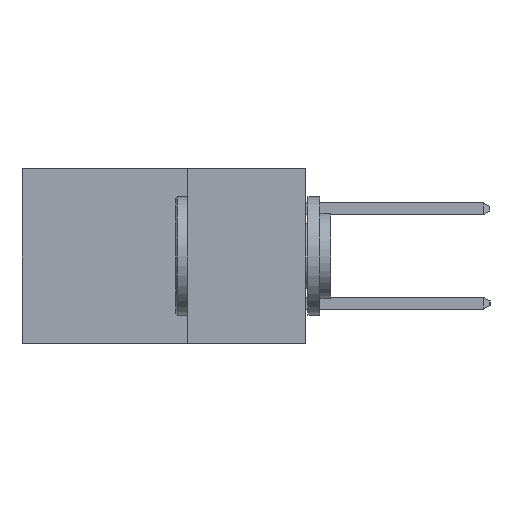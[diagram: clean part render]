
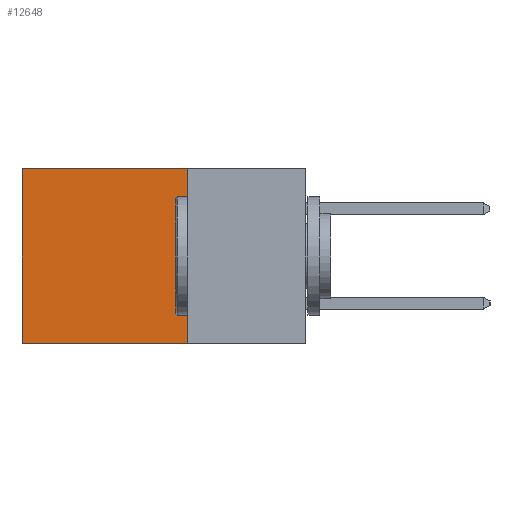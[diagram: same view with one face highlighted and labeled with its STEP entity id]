
A CAD part, left-side view. The second image highlights one B-rep face of the part: STEP entity #12648.
In plain terms, the highlighted planar face has unit normal (-1, 0, 0).
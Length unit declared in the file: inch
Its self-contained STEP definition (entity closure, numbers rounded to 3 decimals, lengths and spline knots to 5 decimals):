
#1976 = CARTESIAN_POINT ( 'NONE',  ( 0.2615, 0.25, -0.37 ) ) ;
#2145 = VECTOR ( 'NONE', #4501, 39.37008 ) ;
#2227 = CARTESIAN_POINT ( 'NONE',  ( 0.2615, 0.25, 0. ) ) ;
#4171 = DIRECTION ( 'NONE',  ( 0., 1., 0. ) ) ;
#4472 = DIRECTION ( 'NONE',  ( 0., 0., -1. ) ) ;
#4501 = DIRECTION ( 'NONE',  ( 0., 0., -1. ) ) ;
#5123 = ORIENTED_EDGE ( 'NONE', *, *, #19356, .T. ) ;
#5946 = VERTEX_POINT ( 'NONE', #17215 ) ;
#6468 = EDGE_CURVE ( 'NONE', #11380, #6584, #14752, .T. ) ;
#6584 = VERTEX_POINT ( 'NONE', #20567 ) ;
#8770 = CARTESIAN_POINT ( 'NONE',  ( 0.2615, 0.25, -0.37 ) ) ;
#9899 = ORIENTED_EDGE ( 'NONE', *, *, #6468, .F. ) ;
#10058 = LINE ( 'NONE', #20970, #2145 ) ;
#10382 = DIRECTION ( 'NONE',  ( 0., 1., 0. ) ) ;
#11293 = AXIS2_PLACEMENT_3D ( 'NONE', #20942, #14453, #4472 ) ;
#11342 = ORIENTED_EDGE ( 'NONE', *, *, #17988, .F. ) ;
#11380 = VERTEX_POINT ( 'NONE', #2227 ) ;
#11642 = VECTOR ( 'NONE', #4171, 39.37008 ) ;
#12648 = ADVANCED_FACE ( 'NONE', ( #15214 ), #17715, .F. ) ;
#13962 = EDGE_CURVE ( 'NONE', #5946, #15379, #10058, .T. ) ;
#14148 = CARTESIAN_POINT ( 'NONE',  ( 0.2615, 0.25, 0. ) ) ;
#14206 = VECTOR ( 'NONE', #17050, 39.37008 ) ;
#14453 = DIRECTION ( 'NONE',  ( 1., 0., 0. ) ) ;
#14752 = LINE ( 'NONE', #8770, #14206 ) ;
#15023 = LINE ( 'NONE', #14148, #11642 ) ;
#15214 = FACE_OUTER_BOUND ( 'NONE', #18525, .T. ) ;
#15379 = VERTEX_POINT ( 'NONE', #18886 ) ;
#17050 = DIRECTION ( 'NONE',  ( 0., 0., -1. ) ) ;
#17167 = LINE ( 'NONE', #1976, #20944 ) ;
#17215 = CARTESIAN_POINT ( 'NONE',  ( 0.2615, 0.6, 0. ) ) ;
#17715 = PLANE ( 'NONE',  #11293 ) ;
#17988 = EDGE_CURVE ( 'NONE', #6584, #15379, #17167, .T. ) ;
#18525 = EDGE_LOOP ( 'NONE', ( #20326, #11342, #9899, #5123 ) ) ;
#18886 = CARTESIAN_POINT ( 'NONE',  ( 0.2615, 0.6, -0.37 ) ) ;
#19356 = EDGE_CURVE ( 'NONE', #11380, #5946, #15023, .T. ) ;
#20326 = ORIENTED_EDGE ( 'NONE', *, *, #13962, .T. ) ;
#20567 = CARTESIAN_POINT ( 'NONE',  ( 0.2615, 0.25, -0.37 ) ) ;
#20942 = CARTESIAN_POINT ( 'NONE',  ( 0.2615, 0.25, -0.37 ) ) ;
#20944 = VECTOR ( 'NONE', #10382, 39.37008 ) ;
#20970 = CARTESIAN_POINT ( 'NONE',  ( 0.2615, 0.6, -0.37 ) ) ;
